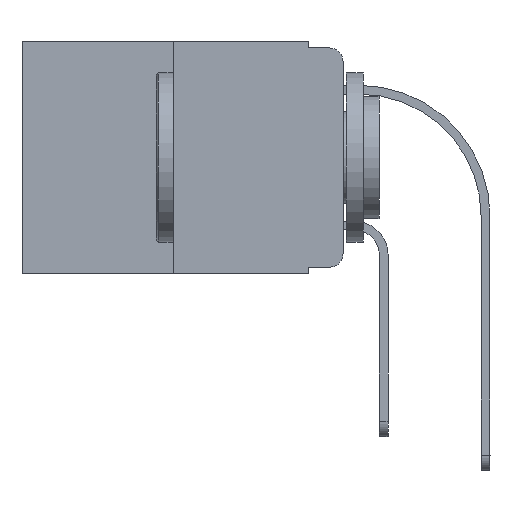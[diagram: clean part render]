
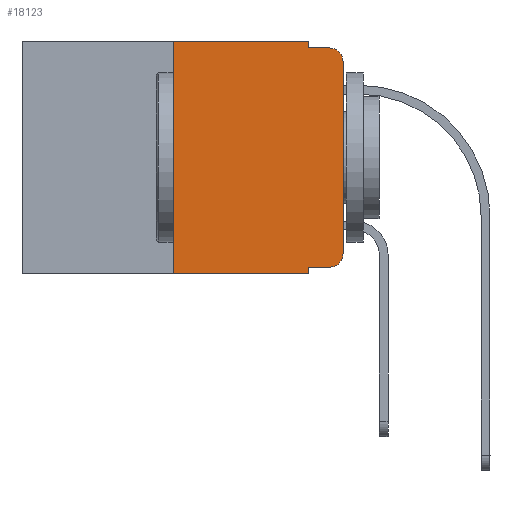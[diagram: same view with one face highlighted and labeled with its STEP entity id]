
A CAD part, left-side view. The second image highlights one B-rep face of the part: STEP entity #18123.
In plain terms, the highlighted planar face has unit normal (-1, 0, 0).
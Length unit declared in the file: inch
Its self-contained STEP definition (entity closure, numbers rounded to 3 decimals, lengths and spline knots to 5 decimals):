
#37 = CARTESIAN_POINT ( 'NONE',  ( 0., 0.02, -0.333 ) ) ;
#166 = CARTESIAN_POINT ( 'NONE',  ( 0., 0.473, 0. ) ) ;
#361 = EDGE_CURVE ( 'NONE', #11619, #18056, #7633, .T. ) ;
#402 = CARTESIAN_POINT ( 'NONE',  ( 0., 0.473, -0.343 ) ) ;
#412 = EDGE_CURVE ( 'NONE', #5242, #14498, #17758, .T. ) ;
#424 = VECTOR ( 'NONE', #1162, 39.37008 ) ;
#573 = ORIENTED_EDGE ( 'NONE', *, *, #412, .F. ) ;
#1076 = DIRECTION ( 'NONE',  ( -1., 0., 0. ) ) ;
#1162 = DIRECTION ( 'NONE',  ( 0., -1., 0. ) ) ;
#1296 = VERTEX_POINT ( 'NONE', #4846 ) ;
#1547 = ORIENTED_EDGE ( 'NONE', *, *, #18002, .F. ) ;
#1555 = VERTEX_POINT ( 'NONE', #7151 ) ;
#2441 = DIRECTION ( 'NONE',  ( 0., 0., -1. ) ) ;
#3317 = FACE_OUTER_BOUND ( 'NONE', #9230, .T. ) ;
#3406 = LINE ( 'NONE', #402, #6889 ) ;
#3410 = DIRECTION ( 'NONE',  ( 0., 0., 1. ) ) ;
#3629 = VERTEX_POINT ( 'NONE', #18480 ) ;
#3805 = DIRECTION ( 'NONE',  ( 1., 0., 0. ) ) ;
#3871 = LINE ( 'NONE', #8236, #11642 ) ;
#3981 = PLANE ( 'NONE',  #13150 ) ;
#4587 = ORIENTED_EDGE ( 'NONE', *, *, #14227, .F. ) ;
#4617 = DIRECTION ( 'NONE',  ( 0., 0., 1. ) ) ;
#4789 = ORIENTED_EDGE ( 'NONE', *, *, #361, .T. ) ;
#4846 = CARTESIAN_POINT ( 'NONE',  ( 0., 0.25, -0.343 ) ) ;
#4877 = VERTEX_POINT ( 'NONE', #14020 ) ;
#5242 = VERTEX_POINT ( 'NONE', #9318 ) ;
#5437 = CARTESIAN_POINT ( 'NONE',  ( 0., 0.051, -0.333 ) ) ;
#5703 = LINE ( 'NONE', #166, #6969 ) ;
#6889 = VECTOR ( 'NONE', #12274, 39.37008 ) ;
#6904 = CARTESIAN_POINT ( 'NONE',  ( 0., 0.02, -0.03 ) ) ;
#6969 = VECTOR ( 'NONE', #19027, 39.37008 ) ;
#7151 = CARTESIAN_POINT ( 'NONE',  ( 0., 0.02, -0.01 ) ) ;
#7633 = LINE ( 'NONE', #17857, #12276 ) ;
#7666 = EDGE_CURVE ( 'NONE', #15351, #11619, #15564, .T. ) ;
#8114 = CARTESIAN_POINT ( 'NONE',  ( 0., 0.02, -0.313 ) ) ;
#8136 = CIRCLE ( 'NONE', #11250, 0.02 ) ;
#8177 = ORIENTED_EDGE ( 'NONE', *, *, #16875, .T. ) ;
#8236 = CARTESIAN_POINT ( 'NONE',  ( 0., 0.051, 0. ) ) ;
#8339 = LINE ( 'NONE', #5437, #424 ) ;
#9026 = VERTEX_POINT ( 'NONE', #17266 ) ;
#9230 = EDGE_LOOP ( 'NONE', ( #4789, #8177, #4587, #11948, #13919, #1547, #18781, #573, #9341, #16137 ) ) ;
#9318 = CARTESIAN_POINT ( 'NONE',  ( 0., 0.051, -0.333 ) ) ;
#9340 = CARTESIAN_POINT ( 'NONE',  ( 0., 0., -0.03 ) ) ;
#9341 = ORIENTED_EDGE ( 'NONE', *, *, #13011, .T. ) ;
#9904 = DIRECTION ( 'NONE',  ( 0., 0., -1. ) ) ;
#10259 = CARTESIAN_POINT ( 'NONE',  ( 0., 0.051, 0. ) ) ;
#10404 = VECTOR ( 'NONE', #16299, 39.37008 ) ;
#10572 = AXIS2_PLACEMENT_3D ( 'NONE', #8114, #18425, #16977 ) ;
#10995 = VECTOR ( 'NONE', #18848, 39.37008 ) ;
#11149 = CARTESIAN_POINT ( 'NONE',  ( 0., 0.051, -0.343 ) ) ;
#11250 = AXIS2_PLACEMENT_3D ( 'NONE', #6904, #1076, #2441 ) ;
#11619 = VERTEX_POINT ( 'NONE', #16386 ) ;
#11642 = VECTOR ( 'NONE', #18542, 39.37008 ) ;
#11665 = LINE ( 'NONE', #12933, #10995 ) ;
#11948 = ORIENTED_EDGE ( 'NONE', *, *, #14478, .F. ) ;
#12274 = DIRECTION ( 'NONE',  ( 0., -1., 0. ) ) ;
#12276 = VECTOR ( 'NONE', #4617, 39.37008 ) ;
#12365 = LINE ( 'NONE', #15189, #14718 ) ;
#12933 = CARTESIAN_POINT ( 'NONE',  ( 0., 0.051, -0.01 ) ) ;
#13011 = EDGE_CURVE ( 'NONE', #5242, #15351, #8339, .T. ) ;
#13150 = AXIS2_PLACEMENT_3D ( 'NONE', #17127, #3805, #9904 ) ;
#13919 = ORIENTED_EDGE ( 'NONE', *, *, #18826, .F. ) ;
#14020 = CARTESIAN_POINT ( 'NONE',  ( 0., 0.25, 0. ) ) ;
#14227 = EDGE_CURVE ( 'NONE', #9026, #1555, #11665, .T. ) ;
#14478 = EDGE_CURVE ( 'NONE', #3629, #9026, #3871, .T. ) ;
#14498 = VERTEX_POINT ( 'NONE', #11149 ) ;
#14718 = VECTOR ( 'NONE', #3410, 39.37008 ) ;
#15189 = CARTESIAN_POINT ( 'NONE',  ( 0., 0.25, 0. ) ) ;
#15351 = VERTEX_POINT ( 'NONE', #37 ) ;
#15564 = CIRCLE ( 'NONE', #10572, 0.02 ) ;
#16137 = ORIENTED_EDGE ( 'NONE', *, *, #7666, .T. ) ;
#16299 = DIRECTION ( 'NONE',  ( 0., 0., -1. ) ) ;
#16386 = CARTESIAN_POINT ( 'NONE',  ( 0., 0., -0.313 ) ) ;
#16716 = EDGE_CURVE ( 'NONE', #1296, #14498, #3406, .T. ) ;
#16875 = EDGE_CURVE ( 'NONE', #18056, #1555, #8136, .T. ) ;
#16977 = DIRECTION ( 'NONE',  ( 0., 0., -1. ) ) ;
#17127 = CARTESIAN_POINT ( 'NONE',  ( 0., 0.473, 0. ) ) ;
#17266 = CARTESIAN_POINT ( 'NONE',  ( 0., 0.051, -0.01 ) ) ;
#17758 = LINE ( 'NONE', #10259, #10404 ) ;
#17857 = CARTESIAN_POINT ( 'NONE',  ( 0., 0., 0. ) ) ;
#18002 = EDGE_CURVE ( 'NONE', #1296, #4877, #12365, .T. ) ;
#18056 = VERTEX_POINT ( 'NONE', #9340 ) ;
#18123 = ADVANCED_FACE ( 'NONE', ( #3317 ), #3981, .F. ) ;
#18425 = DIRECTION ( 'NONE',  ( -1., 0., 0. ) ) ;
#18480 = CARTESIAN_POINT ( 'NONE',  ( 0., 0.051, 0. ) ) ;
#18542 = DIRECTION ( 'NONE',  ( 0., 0., -1. ) ) ;
#18781 = ORIENTED_EDGE ( 'NONE', *, *, #16716, .T. ) ;
#18826 = EDGE_CURVE ( 'NONE', #4877, #3629, #5703, .T. ) ;
#18848 = DIRECTION ( 'NONE',  ( 0., -1., 0. ) ) ;
#19027 = DIRECTION ( 'NONE',  ( 0., -1., 0. ) ) ;
